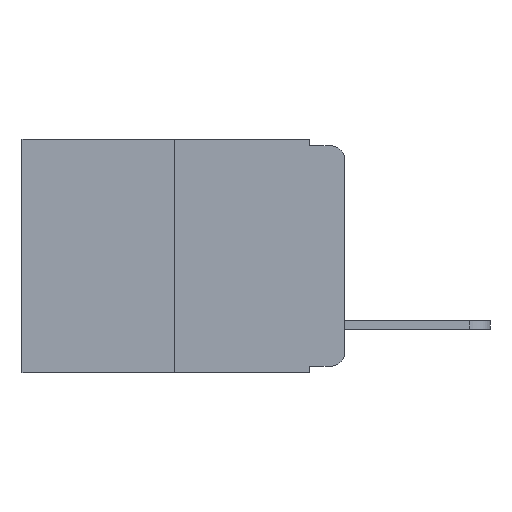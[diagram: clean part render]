
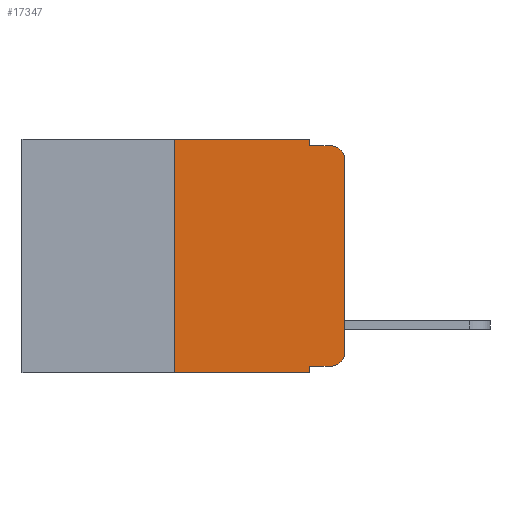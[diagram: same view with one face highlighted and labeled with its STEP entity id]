
A CAD part, left-side view. The second image highlights one B-rep face of the part: STEP entity #17347.
In plain terms, the highlighted planar face has unit normal (-1, 0, 0).
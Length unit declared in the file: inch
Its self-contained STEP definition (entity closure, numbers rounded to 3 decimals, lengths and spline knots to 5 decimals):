
#436 = EDGE_CURVE ( 'NONE', #9995, #23848, #22362, .T. ) ;
#663 = LINE ( 'NONE', #2684, #17104 ) ;
#1042 = EDGE_CURVE ( 'NONE', #10193, #18225, #16817, .T. ) ;
#1076 = LINE ( 'NONE', #23628, #6652 ) ;
#1082 = EDGE_CURVE ( 'NONE', #18225, #10841, #9019, .T. ) ;
#1089 = EDGE_CURVE ( 'NONE', #18693, #10841, #13755, .T. ) ;
#1172 = EDGE_CURVE ( 'NONE', #1917, #18693, #22316, .T. ) ;
#1288 = VERTEX_POINT ( 'NONE', #12226 ) ;
#1352 = EDGE_CURVE ( 'NONE', #9995, #1288, #22591, .T. ) ;
#1357 = EDGE_CURVE ( 'NONE', #6937, #23848, #1076, .T. ) ;
#1547 = EDGE_CURVE ( 'NONE', #6937, #11778, #663, .T. ) ;
#1562 = EDGE_CURVE ( 'NONE', #11778, #10193, #6971, .T. ) ;
#1917 = VERTEX_POINT ( 'NONE', #11046 ) ;
#1929 = DIRECTION ( 'NONE',  ( 0., 0., 1. ) ) ;
#2684 = CARTESIAN_POINT ( 'NONE',  ( 0., 0.051, -0.333 ) ) ;
#4999 = DIRECTION ( 'NONE',  ( 0., -1., 0. ) ) ;
#5330 = CARTESIAN_POINT ( 'NONE',  ( 0., 0.051, -0.343 ) ) ;
#6652 = VECTOR ( 'NONE', #14148, 39.37008 ) ;
#6937 = VERTEX_POINT ( 'NONE', #10159 ) ;
#6971 = CIRCLE ( 'NONE', #16382, 0.02 ) ;
#7690 = DIRECTION ( 'NONE',  ( -1., 0., 0. ) ) ;
#7725 = CARTESIAN_POINT ( 'NONE',  ( 0., 0.02, -0.03 ) ) ;
#7872 = DIRECTION ( 'NONE',  ( 0., 0., -1. ) ) ;
#8345 = VECTOR ( 'NONE', #4999, 39.37008 ) ;
#8974 = DIRECTION ( 'NONE',  ( 0., 0., 1. ) ) ;
#9019 = CIRCLE ( 'NONE', #20519, 0.02 ) ;
#9995 = VERTEX_POINT ( 'NONE', #15445 ) ;
#10159 = CARTESIAN_POINT ( 'NONE',  ( 0., 0.051, -0.333 ) ) ;
#10193 = VERTEX_POINT ( 'NONE', #11595 ) ;
#10841 = VERTEX_POINT ( 'NONE', #23255 ) ;
#11046 = CARTESIAN_POINT ( 'NONE',  ( 0., 0.051, 0. ) ) ;
#11515 = DIRECTION ( 'NONE',  ( 0., -1., 0. ) ) ;
#11595 = CARTESIAN_POINT ( 'NONE',  ( 0., 0., -0.313 ) ) ;
#11778 = VERTEX_POINT ( 'NONE', #15084 ) ;
#11974 = ORIENTED_EDGE ( 'NONE', *, *, #1042, .T. ) ;
#12002 = ORIENTED_EDGE ( 'NONE', *, *, #1082, .T. ) ;
#12226 = CARTESIAN_POINT ( 'NONE',  ( 0., 0.25, 0. ) ) ;
#12400 = ORIENTED_EDGE ( 'NONE', *, *, #1089, .F. ) ;
#12750 = ORIENTED_EDGE ( 'NONE', *, *, #1172, .F. ) ;
#13044 = ORIENTED_EDGE ( 'NONE', *, *, #18902, .F. ) ;
#13189 = ORIENTED_EDGE ( 'NONE', *, *, #1352, .F. ) ;
#13249 = ORIENTED_EDGE ( 'NONE', *, *, #436, .T. ) ;
#13635 = ORIENTED_EDGE ( 'NONE', *, *, #1357, .F. ) ;
#13656 = ORIENTED_EDGE ( 'NONE', *, *, #1547, .T. ) ;
#13673 = CARTESIAN_POINT ( 'NONE',  ( 0., 0.473, 0. ) ) ;
#13755 = LINE ( 'NONE', #22409, #8345 ) ;
#13893 = ORIENTED_EDGE ( 'NONE', *, *, #1562, .T. ) ;
#14148 = DIRECTION ( 'NONE',  ( 0., 0., -1. ) ) ;
#14188 = VECTOR ( 'NONE', #11515, 39.37008 ) ;
#14216 = AXIS2_PLACEMENT_3D ( 'NONE', #16904, #16896, #16873 ) ;
#15084 = CARTESIAN_POINT ( 'NONE',  ( 0., 0.02, -0.333 ) ) ;
#15445 = CARTESIAN_POINT ( 'NONE',  ( 0., 0.25, -0.343 ) ) ;
#15777 = CARTESIAN_POINT ( 'NONE',  ( 0., 0.051, 0. ) ) ;
#16382 = AXIS2_PLACEMENT_3D ( 'NONE', #17910, #17792, #17265 ) ;
#16718 = CARTESIAN_POINT ( 'NONE',  ( 0., 0., -0.03 ) ) ;
#16817 = LINE ( 'NONE', #24244, #24916 ) ;
#16873 = DIRECTION ( 'NONE',  ( 0., 0., -1. ) ) ;
#16896 = DIRECTION ( 'NONE',  ( 1., 0., 0. ) ) ;
#16904 = CARTESIAN_POINT ( 'NONE',  ( 0., 0.473, 0. ) ) ;
#17055 = PLANE ( 'NONE',  #14216 ) ;
#17104 = VECTOR ( 'NONE', #18668, 39.37008 ) ;
#17265 = DIRECTION ( 'NONE',  ( 0., 0., -1. ) ) ;
#17347 = ADVANCED_FACE ( 'NONE', ( #25080 ), #17055, .F. ) ;
#17443 = VECTOR ( 'NONE', #8974, 39.37008 ) ;
#17792 = DIRECTION ( 'NONE',  ( -1., 0., 0. ) ) ;
#17910 = CARTESIAN_POINT ( 'NONE',  ( 0., 0.02, -0.313 ) ) ;
#18225 = VERTEX_POINT ( 'NONE', #16718 ) ;
#18668 = DIRECTION ( 'NONE',  ( 0., -1., 0. ) ) ;
#18693 = VERTEX_POINT ( 'NONE', #21477 ) ;
#18902 = EDGE_CURVE ( 'NONE', #1288, #1917, #19496, .T. ) ;
#19496 = LINE ( 'NONE', #13673, #14188 ) ;
#20519 = AXIS2_PLACEMENT_3D ( 'NONE', #7725, #7690, #22379 ) ;
#21477 = CARTESIAN_POINT ( 'NONE',  ( 0., 0.051, -0.01 ) ) ;
#21772 = VECTOR ( 'NONE', #22662, 39.37008 ) ;
#22316 = LINE ( 'NONE', #15777, #26177 ) ;
#22362 = LINE ( 'NONE', #24918, #21772 ) ;
#22379 = DIRECTION ( 'NONE',  ( 0., 0., -1. ) ) ;
#22409 = CARTESIAN_POINT ( 'NONE',  ( 0., 0.051, -0.01 ) ) ;
#22591 = LINE ( 'NONE', #24902, #17443 ) ;
#22614 = EDGE_LOOP ( 'NONE', ( #11974, #12002, #12400, #12750, #13044, #13189, #13249, #13635, #13656, #13893 ) ) ;
#22662 = DIRECTION ( 'NONE',  ( 0., -1., 0. ) ) ;
#23255 = CARTESIAN_POINT ( 'NONE',  ( 0., 0.02, -0.01 ) ) ;
#23628 = CARTESIAN_POINT ( 'NONE',  ( 0., 0.051, 0. ) ) ;
#23848 = VERTEX_POINT ( 'NONE', #5330 ) ;
#24244 = CARTESIAN_POINT ( 'NONE',  ( 0., 0., 0. ) ) ;
#24902 = CARTESIAN_POINT ( 'NONE',  ( 0., 0.25, 0. ) ) ;
#24916 = VECTOR ( 'NONE', #1929, 39.37008 ) ;
#24918 = CARTESIAN_POINT ( 'NONE',  ( 0., 0.473, -0.343 ) ) ;
#25080 = FACE_OUTER_BOUND ( 'NONE', #22614, .T. ) ;
#26177 = VECTOR ( 'NONE', #7872, 39.37008 ) ;
